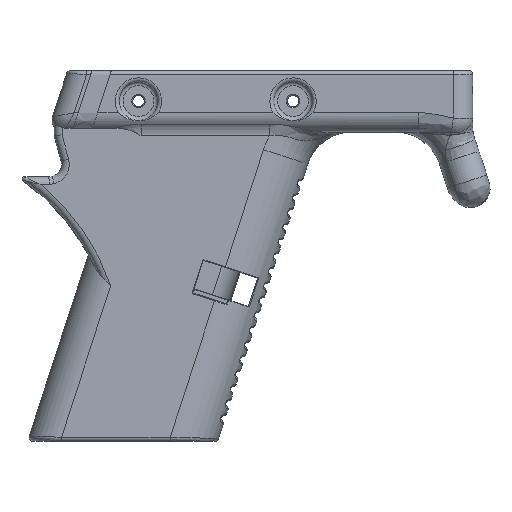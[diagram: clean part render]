
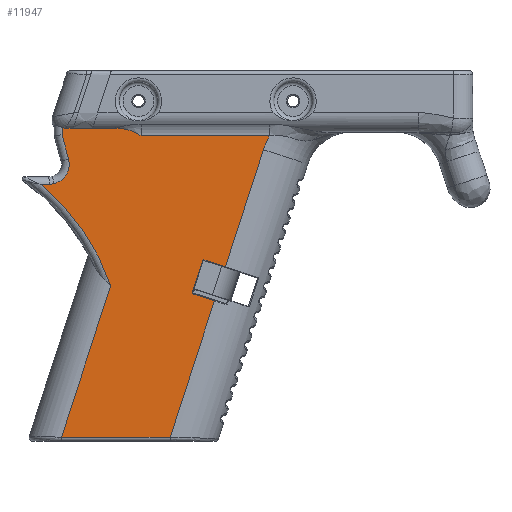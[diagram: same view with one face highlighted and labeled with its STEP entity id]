
A CAD part, top view. The second image highlights one B-rep face of the part: STEP entity #11947.
In plain terms, the highlighted planar face has unit normal (0, 0, 1).
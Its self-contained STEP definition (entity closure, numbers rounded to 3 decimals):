
#641=CIRCLE('',#12744,5.152);
#642=CIRCLE('',#12748,57.942);
#643=CIRCLE('',#12750,0.25);
#644=CIRCLE('',#12751,0.25);
#645=CIRCLE('',#12752,24.);
#1489=FACE_OUTER_BOUND('',#2261,.T.);
#2261=EDGE_LOOP('',(#7957,#7958,#7959,#7960,#7961,#7962,#7963,#7964,#7965,
#7966,#7967,#7968,#7969,#7970,#7971,#7972,#7973,#7974,#7975,#7976,#7977,
#7978));
#3033=B_SPLINE_CURVE_WITH_KNOTS('',3,(#18104,#18105,#18106,#18107,#18108,
#18109,#18110,#18111),.UNSPECIFIED.,.F.,.F.,(4,2,2,4),(-0.515,
-0.363,0.,0.002),.UNSPECIFIED.);
#3034=B_SPLINE_CURVE_WITH_KNOTS('',3,(#18115,#18116,#18117,#18118,#18119,
#18120),.UNSPECIFIED.,.F.,.F.,(4,2,4),(-0.5,-0.25,0.),.UNSPECIFIED.);
#3035=B_SPLINE_CURVE_WITH_KNOTS('',3,(#18123,#18124,#18125,#18126),
 .UNSPECIFIED.,.F.,.F.,(4,4),(-0.105,0.),
 .UNSPECIFIED.);
#3451=LINE('',#18030,#4126);
#3452=LINE('',#18036,#4127);
#3453=LINE('',#18043,#4128);
#3454=LINE('',#18046,#4129);
#3455=LINE('',#18082,#4130);
#3456=LINE('',#18084,#4131);
#3457=LINE('',#18086,#4132);
#3458=LINE('',#18088,#4133);
#3459=LINE('',#18092,#4134);
#3460=LINE('',#18096,#4135);
#3461=LINE('',#18098,#4136);
#3462=LINE('',#18102,#4137);
#3463=LINE('',#18113,#4138);
#3464=LINE('',#18122,#4139);
#4126=VECTOR('',#14142,10.);
#4127=VECTOR('',#14149,10.);
#4128=VECTOR('',#14160,10.);
#4129=VECTOR('',#14163,10.);
#4130=VECTOR('',#14170,10.);
#4131=VECTOR('',#14171,10.);
#4132=VECTOR('',#14172,10.);
#4133=VECTOR('',#14173,10.);
#4134=VECTOR('',#14176,10.);
#4135=VECTOR('',#14179,10.);
#4136=VECTOR('',#14180,10.);
#4137=VECTOR('',#14183,10.);
#4138=VECTOR('',#14184,10.);
#4139=VECTOR('',#14185,10.);
#4813=VERTEX_POINT('',#17995);
#4814=VERTEX_POINT('',#18029);
#4815=VERTEX_POINT('',#18033);
#4816=VERTEX_POINT('',#18035);
#4817=VERTEX_POINT('',#18039);
#4818=VERTEX_POINT('',#18045);
#4819=VERTEX_POINT('',#18068);
#4820=VERTEX_POINT('',#18081);
#4821=VERTEX_POINT('',#18083);
#4822=VERTEX_POINT('',#18085);
#4823=VERTEX_POINT('',#18087);
#4824=VERTEX_POINT('',#18089);
#4825=VERTEX_POINT('',#18091);
#4826=VERTEX_POINT('',#18093);
#4827=VERTEX_POINT('',#18095);
#4828=VERTEX_POINT('',#18097);
#4829=VERTEX_POINT('',#18099);
#4830=VERTEX_POINT('',#18101);
#4831=VERTEX_POINT('',#18103);
#4832=VERTEX_POINT('',#18112);
#4833=VERTEX_POINT('',#18114);
#4834=VERTEX_POINT('',#18121);
#5980=EDGE_CURVE('',#4813,#4814,#3451,.T.);
#5983=EDGE_CURVE('',#4815,#4816,#3452,.T.);
#5986=EDGE_CURVE('',#4817,#4815,#641,.T.);
#5987=EDGE_CURVE('',#4814,#4817,#3453,.T.);
#5988=EDGE_CURVE('',#4816,#4818,#3454,.T.);
#5991=EDGE_CURVE('',#4819,#4813,#642,.T.);
#5992=EDGE_CURVE('',#4820,#4819,#3455,.T.);
#5993=EDGE_CURVE('',#4821,#4820,#3456,.T.);
#5994=EDGE_CURVE('',#4822,#4821,#3457,.T.);
#5995=EDGE_CURVE('',#4823,#4822,#3458,.T.);
#5996=EDGE_CURVE('',#4824,#4823,#643,.T.);
#5997=EDGE_CURVE('',#4825,#4824,#3459,.T.);
#5998=EDGE_CURVE('',#4826,#4825,#644,.T.);
#5999=EDGE_CURVE('',#4827,#4826,#3460,.T.);
#6000=EDGE_CURVE('',#4828,#4827,#3461,.T.);
#6001=EDGE_CURVE('',#4829,#4828,#645,.T.);
#6002=EDGE_CURVE('',#4830,#4829,#3462,.T.);
#6003=EDGE_CURVE('',#4831,#4830,#3033,.T.);
#6004=EDGE_CURVE('',#4832,#4831,#3463,.T.);
#6005=EDGE_CURVE('',#4833,#4832,#3034,.T.);
#6006=EDGE_CURVE('',#4834,#4833,#3464,.T.);
#6007=EDGE_CURVE('',#4818,#4834,#3035,.T.);
#7957=ORIENTED_EDGE('',*,*,#5988,.F.);
#7958=ORIENTED_EDGE('',*,*,#5983,.F.);
#7959=ORIENTED_EDGE('',*,*,#5986,.F.);
#7960=ORIENTED_EDGE('',*,*,#5987,.F.);
#7961=ORIENTED_EDGE('',*,*,#5980,.F.);
#7962=ORIENTED_EDGE('',*,*,#5991,.F.);
#7963=ORIENTED_EDGE('',*,*,#5992,.F.);
#7964=ORIENTED_EDGE('',*,*,#5993,.F.);
#7965=ORIENTED_EDGE('',*,*,#5994,.F.);
#7966=ORIENTED_EDGE('',*,*,#5995,.F.);
#7967=ORIENTED_EDGE('',*,*,#5996,.F.);
#7968=ORIENTED_EDGE('',*,*,#5997,.F.);
#7969=ORIENTED_EDGE('',*,*,#5998,.F.);
#7970=ORIENTED_EDGE('',*,*,#5999,.F.);
#7971=ORIENTED_EDGE('',*,*,#6000,.F.);
#7972=ORIENTED_EDGE('',*,*,#6001,.F.);
#7973=ORIENTED_EDGE('',*,*,#6002,.F.);
#7974=ORIENTED_EDGE('',*,*,#6003,.F.);
#7975=ORIENTED_EDGE('',*,*,#6004,.F.);
#7976=ORIENTED_EDGE('',*,*,#6005,.F.);
#7977=ORIENTED_EDGE('',*,*,#6006,.F.);
#7978=ORIENTED_EDGE('',*,*,#6007,.F.);
#11757=PLANE('',#12749);
#11947=ADVANCED_FACE('',(#1489),#11757,.T.);
#12744=AXIS2_PLACEMENT_3D('',#18041,#14156,#14157);
#12748=AXIS2_PLACEMENT_3D('',#18079,#14166,#14167);
#12749=AXIS2_PLACEMENT_3D('',#18080,#14168,#14169);
#12750=AXIS2_PLACEMENT_3D('',#18090,#14174,#14175);
#12751=AXIS2_PLACEMENT_3D('',#18094,#14177,#14178);
#12752=AXIS2_PLACEMENT_3D('',#18100,#14181,#14182);
#14142=DIRECTION('',(1.,0.,0.));
#14149=DIRECTION('',(-0.259,0.966,0.));
#14156=DIRECTION('center_axis',(0.,0.,1.));
#14157=DIRECTION('ref_axis',(0.858,-0.513,0.));
#14160=DIRECTION('',(0.973,0.23,0.));
#14163=DIRECTION('',(0.,1.,0.));
#14166=DIRECTION('center_axis',(0.,0.,1.));
#14167=DIRECTION('ref_axis',(0.816,0.579,0.));
#14168=DIRECTION('center_axis',(0.,0.,1.));
#14169=DIRECTION('ref_axis',(1.,0.,0.));
#14170=DIRECTION('',(0.309,0.951,0.));
#14171=DIRECTION('',(-1.,0.,0.));
#14172=DIRECTION('',(-0.309,-0.951,0.));
#14173=DIRECTION('',(0.951,-0.309,0.));
#14174=DIRECTION('center_axis',(0.,0.,1.));
#14175=DIRECTION('ref_axis',(-0.891,-0.454,0.));
#14176=DIRECTION('',(-0.309,-0.951,0.));
#14177=DIRECTION('center_axis',(0.,0.,1.));
#14178=DIRECTION('ref_axis',(-0.454,0.891,0.));
#14179=DIRECTION('',(-0.951,0.309,0.));
#14180=DIRECTION('',(-0.309,-0.951,0.));
#14181=DIRECTION('center_axis',(0.,0.,1.));
#14182=DIRECTION('ref_axis',(-0.588,0.809,0.));
#14183=DIRECTION('',(1.,0.,0.));
#14184=DIRECTION('',(1.,0.,0.));
#14185=DIRECTION('',(1.,0.,0.));
#17995=CARTESIAN_POINT('',(112.326,-48.283,14.011));
#18029=CARTESIAN_POINT('',(114.54,-48.283,14.011));
#18030=CARTESIAN_POINT('',(130.371,-48.283,14.011));
#18033=CARTESIAN_POINT('',(119.45,-41.67,14.011));
#18035=CARTESIAN_POINT('',(117.761,-35.373,14.011));
#18036=CARTESIAN_POINT('',(123.6,-57.147,14.011));
#18039=CARTESIAN_POINT('',(115.657,-48.019,14.011));
#18041=CARTESIAN_POINT('Origin',(114.474,-43.005,14.011));
#18043=CARTESIAN_POINT('',(127.257,-45.28,14.011));
#18045=CARTESIAN_POINT('',(117.761,-33.468,14.011));
#18046=CARTESIAN_POINT('',(117.761,-55.136,14.011));
#18068=CARTESIAN_POINT('',(130.334,-74.432,14.011));
#18079=CARTESIAN_POINT('Origin',(75.436,-92.964,14.011));
#18080=CARTESIAN_POINT('Origin',(146.434,-74.636,14.011));
#18081=CARTESIAN_POINT('',(117.596,-113.636,14.011));
#18082=CARTESIAN_POINT('',(137.136,-53.497,14.011));
#18083=CARTESIAN_POINT('',(145.723,-113.636,14.011));
#18084=CARTESIAN_POINT('',(127.647,-113.636,14.011));
#18085=CARTESIAN_POINT('',(157.184,-78.362,14.011));
#18086=CARTESIAN_POINT('',(151.927,-94.54,14.011));
#18087=CARTESIAN_POINT('',(151.621,-76.555,14.011));
#18088=CARTESIAN_POINT('',(153.344,-77.115,14.011));
#18089=CARTESIAN_POINT('',(151.461,-76.24,14.011));
#18090=CARTESIAN_POINT('Origin',(151.698,-76.317,14.011));
#18091=CARTESIAN_POINT('',(154.163,-67.921,14.011));
#18092=CARTESIAN_POINT('',(152.827,-72.035,14.011));
#18093=CARTESIAN_POINT('',(154.479,-67.761,14.011));
#18094=CARTESIAN_POINT('Origin',(154.401,-67.998,14.011));
#18095=CARTESIAN_POINT('',(160.041,-69.568,14.011));
#18096=CARTESIAN_POINT('',(156.534,-68.429,14.011));
#18097=CARTESIAN_POINT('',(169.902,-39.22,14.011));
#18098=CARTESIAN_POINT('',(151.927,-94.54,14.011));
#18099=CARTESIAN_POINT('',(171.397,-35.636,14.011));
#18100=CARTESIAN_POINT('Origin',(192.727,-46.636,14.011));
#18101=CARTESIAN_POINT('',(138.229,-35.636,14.011));
#18102=CARTESIAN_POINT('',(129.031,-35.636,14.011));
#18103=CARTESIAN_POINT('',(131.409,-33.636,14.011));
#18104=CARTESIAN_POINT('Ctrl Pts',(131.41,-33.636,14.011));
#18105=CARTESIAN_POINT('Ctrl Pts',(132.738,-33.634,14.011));
#18106=CARTESIAN_POINT('Ctrl Pts',(133.767,-33.825,14.011));
#18107=CARTESIAN_POINT('Ctrl Pts',(135.991,-34.352,14.011));
#18108=CARTESIAN_POINT('Ctrl Pts',(137.204,-34.957,14.011));
#18109=CARTESIAN_POINT('Ctrl Pts',(138.218,-35.629,14.011));
#18110=CARTESIAN_POINT('Ctrl Pts',(138.223,-35.633,14.011));
#18111=CARTESIAN_POINT('Ctrl Pts',(138.229,-35.636,14.011));
#18112=CARTESIAN_POINT('',(125.665,-33.636,14.011));
#18113=CARTESIAN_POINT('',(134.031,-33.636,14.011));
#18114=CARTESIAN_POINT('',(120.665,-33.636,14.011));
#18115=CARTESIAN_POINT('Ctrl Pts',(120.665,-33.636,14.011));
#18116=CARTESIAN_POINT('Ctrl Pts',(121.498,-33.636,14.011));
#18117=CARTESIAN_POINT('Ctrl Pts',(122.331,-33.636,14.011));
#18118=CARTESIAN_POINT('Ctrl Pts',(123.998,-33.636,14.011));
#18119=CARTESIAN_POINT('Ctrl Pts',(124.831,-33.636,14.011));
#18120=CARTESIAN_POINT('Ctrl Pts',(125.665,-33.636,14.011));
#18121=CARTESIAN_POINT('',(118.711,-33.636,14.011));
#18122=CARTESIAN_POINT('',(129.031,-33.636,14.011));
#18123=CARTESIAN_POINT('Ctrl Pts',(117.761,-33.468,14.011));
#18124=CARTESIAN_POINT('Ctrl Pts',(118.042,-33.574,14.011));
#18125=CARTESIAN_POINT('Ctrl Pts',(118.361,-33.636,14.011));
#18126=CARTESIAN_POINT('Ctrl Pts',(118.711,-33.636,14.011));
